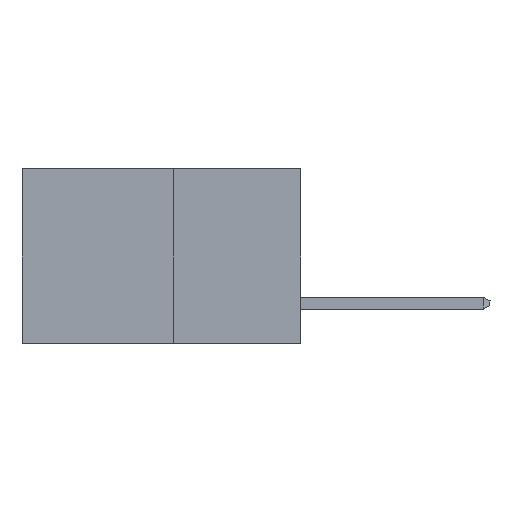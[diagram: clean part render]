
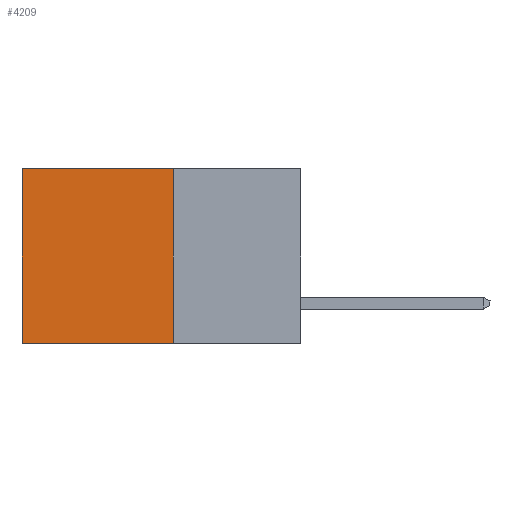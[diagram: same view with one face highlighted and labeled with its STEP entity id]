
A CAD part, left-side view. The second image highlights one B-rep face of the part: STEP entity #4209.
In plain terms, the highlighted planar face has unit normal (-1, 0, 0).
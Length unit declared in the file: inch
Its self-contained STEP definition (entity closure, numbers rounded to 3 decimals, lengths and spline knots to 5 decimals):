
#346 = VECTOR ( 'NONE', #702, 39.37008 ) ;
#388 = VERTEX_POINT ( 'NONE', #5068 ) ;
#702 = DIRECTION ( 'NONE',  ( 0., 1., 0. ) ) ;
#834 = CARTESIAN_POINT ( 'NONE',  ( 0.277, 0.27, -0.37 ) ) ;
#1188 = CARTESIAN_POINT ( 'NONE',  ( 0.277, 0.27, -0.37 ) ) ;
#1212 = ORIENTED_EDGE ( 'NONE', *, *, #8670, .T. ) ;
#1265 = DIRECTION ( 'NONE',  ( 0., 0., -1. ) ) ;
#1307 = DIRECTION ( 'NONE',  ( 1., 0., 0. ) ) ;
#1610 = DIRECTION ( 'NONE',  ( 0., 0., -1. ) ) ;
#1780 = ORIENTED_EDGE ( 'NONE', *, *, #9058, .F. ) ;
#1788 = DIRECTION ( 'NONE',  ( 0., 1., 0. ) ) ;
#2051 = FACE_OUTER_BOUND ( 'NONE', #8769, .T. ) ;
#2109 = VERTEX_POINT ( 'NONE', #4721 ) ;
#3199 = AXIS2_PLACEMENT_3D ( 'NONE', #7602, #1307, #1265 ) ;
#4103 = VERTEX_POINT ( 'NONE', #8092 ) ;
#4209 = ADVANCED_FACE ( 'NONE', ( #2051 ), #7520, .F. ) ;
#4321 = VECTOR ( 'NONE', #1610, 39.37008 ) ;
#4494 = ORIENTED_EDGE ( 'NONE', *, *, #7099, .T. ) ;
#4542 = CARTESIAN_POINT ( 'NONE',  ( 0.277, 0.59, -0.37 ) ) ;
#4580 = LINE ( 'NONE', #9909, #4321 ) ;
#4721 = CARTESIAN_POINT ( 'NONE',  ( 0.277, 0.59, -0.37 ) ) ;
#5068 = CARTESIAN_POINT ( 'NONE',  ( 0.277, 0.27, 0. ) ) ;
#5072 = EDGE_CURVE ( 'NONE', #9500, #2109, #6765, .T. ) ;
#6433 = LINE ( 'NONE', #6995, #8372 ) ;
#6708 = LINE ( 'NONE', #4542, #8621 ) ;
#6765 = LINE ( 'NONE', #1188, #346 ) ;
#6995 = CARTESIAN_POINT ( 'NONE',  ( 0.277, 0.27, 0. ) ) ;
#7099 = EDGE_CURVE ( 'NONE', #4103, #2109, #6708, .T. ) ;
#7520 = PLANE ( 'NONE',  #3199 ) ;
#7602 = CARTESIAN_POINT ( 'NONE',  ( 0.277, 0.27, -0.37 ) ) ;
#8092 = CARTESIAN_POINT ( 'NONE',  ( 0.277, 0.59, 0. ) ) ;
#8372 = VECTOR ( 'NONE', #1788, 39.37008 ) ;
#8621 = VECTOR ( 'NONE', #9122, 39.37008 ) ;
#8670 = EDGE_CURVE ( 'NONE', #388, #4103, #6433, .T. ) ;
#8769 = EDGE_LOOP ( 'NONE', ( #4494, #8906, #1780, #1212 ) ) ;
#8906 = ORIENTED_EDGE ( 'NONE', *, *, #5072, .F. ) ;
#9058 = EDGE_CURVE ( 'NONE', #388, #9500, #4580, .T. ) ;
#9122 = DIRECTION ( 'NONE',  ( 0., 0., -1. ) ) ;
#9500 = VERTEX_POINT ( 'NONE', #834 ) ;
#9909 = CARTESIAN_POINT ( 'NONE',  ( 0.277, 0.27, -0.37 ) ) ;
